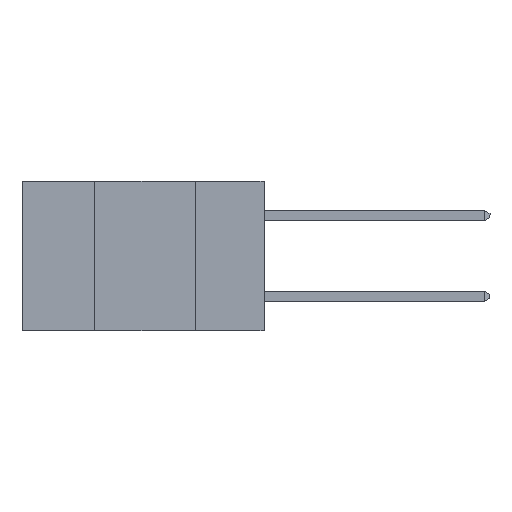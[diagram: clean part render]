
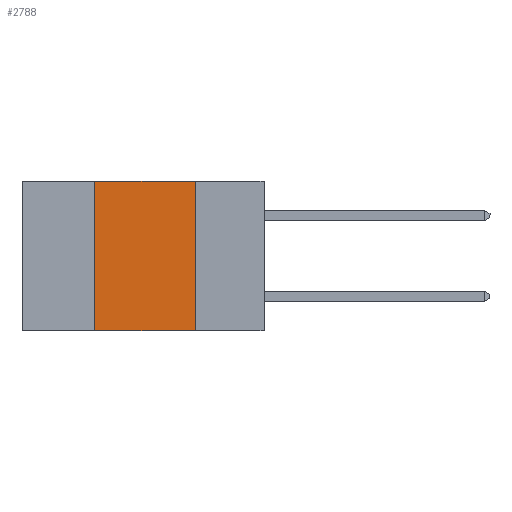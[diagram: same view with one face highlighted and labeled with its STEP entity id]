
A CAD part, left-side view. The second image highlights one B-rep face of the part: STEP entity #2788.
In plain terms, the highlighted planar face has unit normal (-1, 0, 0).
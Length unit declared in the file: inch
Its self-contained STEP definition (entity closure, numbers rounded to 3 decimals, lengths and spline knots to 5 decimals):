
#324 = LINE ( 'NONE', #3246, #6027 ) ;
#535 = ORIENTED_EDGE ( 'NONE', *, *, #11912, .F. ) ;
#578 = PLANE ( 'NONE',  #14201 ) ;
#1657 = LINE ( 'NONE', #14020, #13374 ) ;
#2149 = VERTEX_POINT ( 'NONE', #3092 ) ;
#2788 = ADVANCED_FACE ( 'NONE', ( #10767 ), #578, .F. ) ;
#3092 = CARTESIAN_POINT ( 'NONE',  ( 0., 0.42, 0. ) ) ;
#3246 = CARTESIAN_POINT ( 'NONE',  ( 0., 0.6, -0.37 ) ) ;
#3561 = ORIENTED_EDGE ( 'NONE', *, *, #4138, .F. ) ;
#3977 = VERTEX_POINT ( 'NONE', #11068 ) ;
#4138 = EDGE_CURVE ( 'NONE', #3977, #2149, #12950, .T. ) ;
#4667 = VERTEX_POINT ( 'NONE', #14648 ) ;
#5086 = DIRECTION ( 'NONE',  ( 0., 0., -1. ) ) ;
#5537 = DIRECTION ( 'NONE',  ( 0., -1., 0. ) ) ;
#6027 = VECTOR ( 'NONE', #12503, 39.37008 ) ;
#6314 = EDGE_CURVE ( 'NONE', #8380, #4667, #1657, .T. ) ;
#6332 = DIRECTION ( 'NONE',  ( 0., 0., 1. ) ) ;
#6502 = LINE ( 'NONE', #14497, #12306 ) ;
#6863 = ORIENTED_EDGE ( 'NONE', *, *, #11267, .T. ) ;
#8380 = VERTEX_POINT ( 'NONE', #8930 ) ;
#8930 = CARTESIAN_POINT ( 'NONE',  ( 0., 0.17, 0. ) ) ;
#9008 = CARTESIAN_POINT ( 'NONE',  ( 0., 0.42, 0. ) ) ;
#9577 = DIRECTION ( 'NONE',  ( 0., 0., -1. ) ) ;
#10159 = VECTOR ( 'NONE', #6332, 39.37008 ) ;
#10176 = DIRECTION ( 'NONE',  ( 1., 0., 0. ) ) ;
#10767 = FACE_OUTER_BOUND ( 'NONE', #13602, .T. ) ;
#11068 = CARTESIAN_POINT ( 'NONE',  ( 0., 0.42, -0.37 ) ) ;
#11267 = EDGE_CURVE ( 'NONE', #3977, #4667, #324, .T. ) ;
#11912 = EDGE_CURVE ( 'NONE', #2149, #8380, #6502, .T. ) ;
#11975 = ORIENTED_EDGE ( 'NONE', *, *, #6314, .F. ) ;
#12097 = CARTESIAN_POINT ( 'NONE',  ( 0., 0.6, 0. ) ) ;
#12306 = VECTOR ( 'NONE', #5537, 39.37008 ) ;
#12503 = DIRECTION ( 'NONE',  ( 0., -1., 0. ) ) ;
#12950 = LINE ( 'NONE', #9008, #10159 ) ;
#13374 = VECTOR ( 'NONE', #5086, 39.37008 ) ;
#13602 = EDGE_LOOP ( 'NONE', ( #11975, #535, #3561, #6863 ) ) ;
#14020 = CARTESIAN_POINT ( 'NONE',  ( 0., 0.17, 0. ) ) ;
#14201 = AXIS2_PLACEMENT_3D ( 'NONE', #12097, #10176, #9577 ) ;
#14497 = CARTESIAN_POINT ( 'NONE',  ( 0., 0.6, 0. ) ) ;
#14648 = CARTESIAN_POINT ( 'NONE',  ( 0., 0.17, -0.37 ) ) ;
